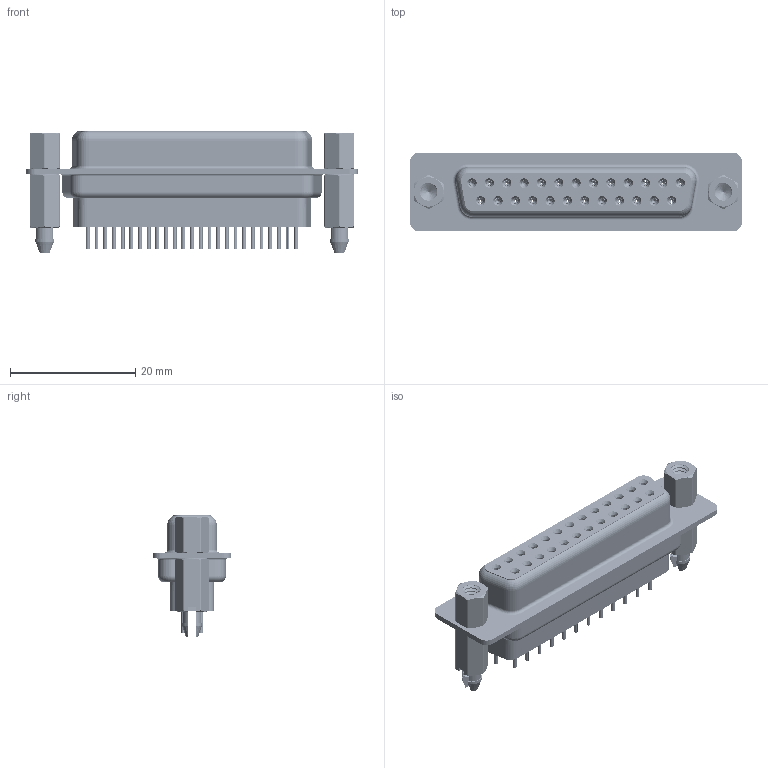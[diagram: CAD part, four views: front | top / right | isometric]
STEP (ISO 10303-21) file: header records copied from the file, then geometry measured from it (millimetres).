
FILE_DESCRIPTION (( 'STEP AP203' ), '1' );
FILE_NAME ('628-025-228-267.STEP', '2020-07-21T13:38:22', ( '' ), ( '' ), 'SwSTEP 2.0', 'SolidWorks 2020', '' );
FILE_SCHEMA (( 'CONFIG_CONTROL_DESIGN' ));
Length unit declared in the file: millimetre
Products named in the file (8): 628 Contact Row 1_28L; 628 4-40 Threaded Boardlock_FF; 628 Contact Row 2_28L; 628 Shell Front_25 Contacts; 628 Shell Rear_25 Contacts; 628 4-40 Hex Standoff; 628 Housing_25 FF; 628-025-228-267
Assembly tree (32 placements, depth 2):
  628-025-228-267
    628 Housing_25 FF
    628 Shell Front_25 Contacts
    628 Shell Rear_25 Contacts
    628 Contact Row 1_28L  x13
    628 Contact Row 2_28L  x12
    628 4-40 Hex Standoff  x2
    628 4-40 Threaded Boardlock_FF  x2
Bounding box: 53 x 12.6 x 19.4 mm (x, y, z)
Volume: 4815.9 mm3; surface area: 11416 mm2
Topology: 33 solids, 33 shells, 3797 faces, 9782 edges, 6110 vertices
Faces by surface type: cylinder 1155, plane 902, torus 713, bspline 566, cone 461
Entity records: 51179 total; most frequent: CARTESIAN_POINT 26061, DIRECTION 4996, ORIENTED_EDGE 4942, EDGE_CURVE 2471, AXIS2_PLACEMENT_3D 2063, VERTEX_POINT 1575, EDGE_LOOP 1196, CIRCLE 1104
